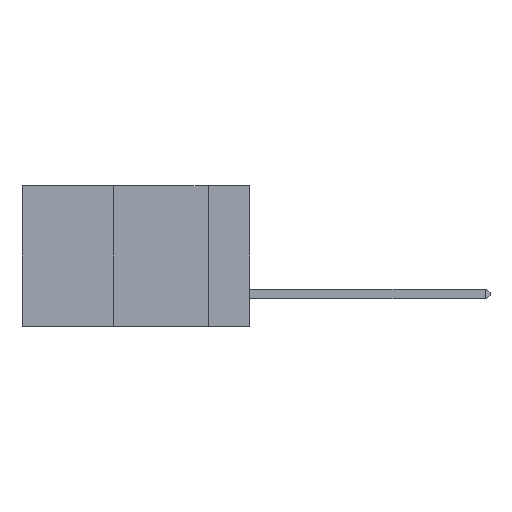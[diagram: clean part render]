
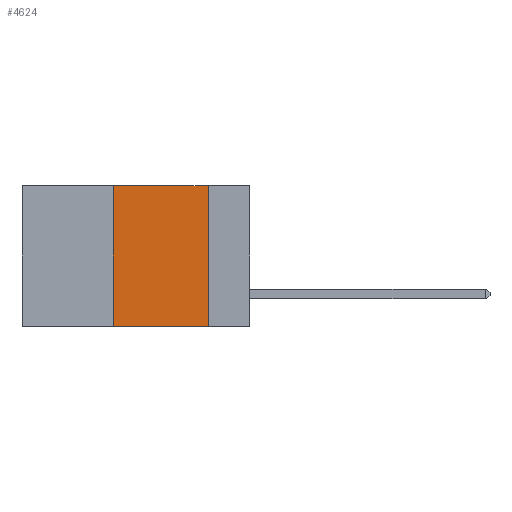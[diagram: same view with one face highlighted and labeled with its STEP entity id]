
A CAD part, left-side view. The second image highlights one B-rep face of the part: STEP entity #4624.
In plain terms, the highlighted planar face has unit normal (-1, 0, 0).
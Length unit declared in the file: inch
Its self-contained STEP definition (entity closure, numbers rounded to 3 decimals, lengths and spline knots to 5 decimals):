
#161 = VERTEX_POINT ( 'NONE', #4790 ) ;
#188 = VECTOR ( 'NONE', #5505, 39.37008 ) ;
#370 = VECTOR ( 'NONE', #2113, 39.37008 ) ;
#559 = ORIENTED_EDGE ( 'NONE', *, *, #5766, .F. ) ;
#1134 = CARTESIAN_POINT ( 'NONE',  ( 0., 0.36, 0. ) ) ;
#1709 = DIRECTION ( 'NONE',  ( 0., 0., -1. ) ) ;
#2113 = DIRECTION ( 'NONE',  ( 0., 0., 1. ) ) ;
#3628 = EDGE_CURVE ( 'NONE', #11350, #161, #11605, .T. ) ;
#3783 = CARTESIAN_POINT ( 'NONE',  ( 0., 0.6, -0.37 ) ) ;
#4624 = ADVANCED_FACE ( 'NONE', ( #9232 ), #8241, .F. ) ;
#4790 = CARTESIAN_POINT ( 'NONE',  ( 0., 0.11, -0.37 ) ) ;
#5505 = DIRECTION ( 'NONE',  ( 0., 0., -1. ) ) ;
#5559 = CARTESIAN_POINT ( 'NONE',  ( 0., 0.11, 0. ) ) ;
#5570 = CARTESIAN_POINT ( 'NONE',  ( 0., 0.6, 0. ) ) ;
#5716 = ORIENTED_EDGE ( 'NONE', *, *, #3628, .F. ) ;
#5766 = EDGE_CURVE ( 'NONE', #9437, #11350, #11333, .T. ) ;
#6568 = VECTOR ( 'NONE', #8396, 39.37008 ) ;
#6651 = VECTOR ( 'NONE', #9035, 39.37008 ) ;
#6716 = CARTESIAN_POINT ( 'NONE',  ( 0., 0.36, -0.37 ) ) ;
#7146 = LINE ( 'NONE', #3783, #6568 ) ;
#7379 = DIRECTION ( 'NONE',  ( 1., 0., 0. ) ) ;
#7932 = LINE ( 'NONE', #1134, #370 ) ;
#8046 = VERTEX_POINT ( 'NONE', #6716 ) ;
#8104 = CARTESIAN_POINT ( 'NONE',  ( 0., 0.6, 0. ) ) ;
#8241 = PLANE ( 'NONE',  #8585 ) ;
#8396 = DIRECTION ( 'NONE',  ( 0., -1., 0. ) ) ;
#8585 = AXIS2_PLACEMENT_3D ( 'NONE', #5570, #7379, #1709 ) ;
#9035 = DIRECTION ( 'NONE',  ( 0., -1., 0. ) ) ;
#9232 = FACE_OUTER_BOUND ( 'NONE', #11698, .T. ) ;
#9366 = ORIENTED_EDGE ( 'NONE', *, *, #10591, .F. ) ;
#9437 = VERTEX_POINT ( 'NONE', #10411 ) ;
#9854 = EDGE_CURVE ( 'NONE', #8046, #161, #7146, .T. ) ;
#10411 = CARTESIAN_POINT ( 'NONE',  ( 0., 0.36, 0. ) ) ;
#10591 = EDGE_CURVE ( 'NONE', #8046, #9437, #7932, .T. ) ;
#10677 = CARTESIAN_POINT ( 'NONE',  ( 0., 0.11, 0. ) ) ;
#11333 = LINE ( 'NONE', #8104, #6651 ) ;
#11350 = VERTEX_POINT ( 'NONE', #10677 ) ;
#11605 = LINE ( 'NONE', #5559, #188 ) ;
#11647 = ORIENTED_EDGE ( 'NONE', *, *, #9854, .T. ) ;
#11698 = EDGE_LOOP ( 'NONE', ( #5716, #559, #9366, #11647 ) ) ;
